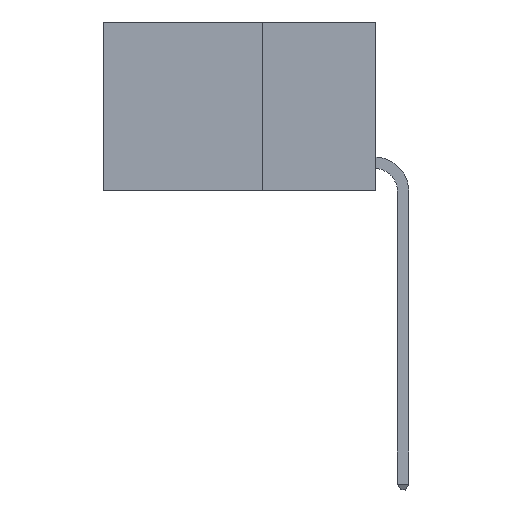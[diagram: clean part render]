
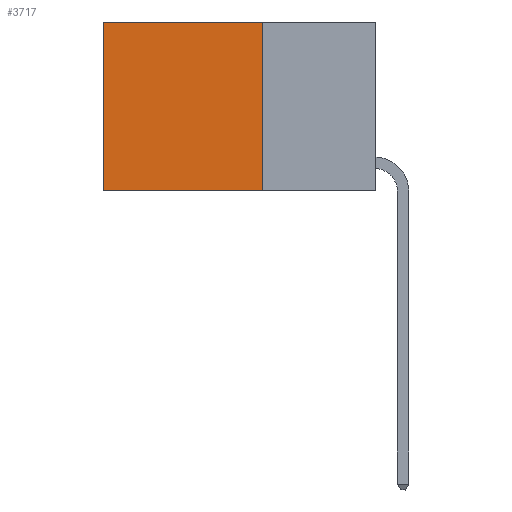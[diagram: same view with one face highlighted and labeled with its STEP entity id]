
A CAD part, left-side view. The second image highlights one B-rep face of the part: STEP entity #3717.
In plain terms, the highlighted planar face has unit normal (-1, 0, 0).
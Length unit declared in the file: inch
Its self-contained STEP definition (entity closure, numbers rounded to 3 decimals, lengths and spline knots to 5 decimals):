
#751 = VECTOR ( 'NONE', #4955, 39.37008 ) ;
#864 = LINE ( 'NONE', #11649, #14065 ) ;
#1375 = DIRECTION ( 'NONE',  ( 0., 0., -1. ) ) ;
#2214 = ORIENTED_EDGE ( 'NONE', *, *, #13067, .T. ) ;
#3605 = DIRECTION ( 'NONE',  ( 0., 0., -1. ) ) ;
#3717 = ADVANCED_FACE ( 'NONE', ( #18977 ), #9644, .F. ) ;
#4151 = CARTESIAN_POINT ( 'NONE',  ( 0.2625, 0.25, -0.37 ) ) ;
#4367 = DIRECTION ( 'NONE',  ( 0., 0., -1. ) ) ;
#4724 = EDGE_LOOP ( 'NONE', ( #7976, #12554, #18352, #2214 ) ) ;
#4955 = DIRECTION ( 'NONE',  ( 0., 1., 0. ) ) ;
#5164 = LINE ( 'NONE', #11529, #751 ) ;
#5405 = AXIS2_PLACEMENT_3D ( 'NONE', #7974, #11284, #1375 ) ;
#5877 = CARTESIAN_POINT ( 'NONE',  ( 0.2625, 0.25, 0. ) ) ;
#7974 = CARTESIAN_POINT ( 'NONE',  ( 0.2625, 0.25, 0. ) ) ;
#7976 = ORIENTED_EDGE ( 'NONE', *, *, #19642, .T. ) ;
#9078 = EDGE_CURVE ( 'NONE', #11327, #13125, #5164, .T. ) ;
#9644 = PLANE ( 'NONE',  #5405 ) ;
#11284 = DIRECTION ( 'NONE',  ( 1., 0., 0. ) ) ;
#11327 = VERTEX_POINT ( 'NONE', #4151 ) ;
#11359 = VERTEX_POINT ( 'NONE', #5877 ) ;
#11529 = CARTESIAN_POINT ( 'NONE',  ( 0.2625, 0.25, -0.37 ) ) ;
#11649 = CARTESIAN_POINT ( 'NONE',  ( 0.2625, 0.25, 0. ) ) ;
#11789 = CARTESIAN_POINT ( 'NONE',  ( 0.2625, 0.6, -0.37 ) ) ;
#12554 = ORIENTED_EDGE ( 'NONE', *, *, #9078, .F. ) ;
#12789 = CARTESIAN_POINT ( 'NONE',  ( 0.2625, 0.6, 0. ) ) ;
#13067 = EDGE_CURVE ( 'NONE', #11359, #14006, #864, .T. ) ;
#13125 = VERTEX_POINT ( 'NONE', #11789 ) ;
#13495 = CARTESIAN_POINT ( 'NONE',  ( 0.2625, 0.6, 0. ) ) ;
#14006 = VERTEX_POINT ( 'NONE', #12789 ) ;
#14065 = VECTOR ( 'NONE', #18256, 39.37008 ) ;
#17472 = CARTESIAN_POINT ( 'NONE',  ( 0.2625, 0.25, 0. ) ) ;
#17619 = LINE ( 'NONE', #13495, #18124 ) ;
#18124 = VECTOR ( 'NONE', #3605, 39.37008 ) ;
#18256 = DIRECTION ( 'NONE',  ( 0., 1., 0. ) ) ;
#18352 = ORIENTED_EDGE ( 'NONE', *, *, #18653, .F. ) ;
#18653 = EDGE_CURVE ( 'NONE', #11359, #11327, #20743, .T. ) ;
#18977 = FACE_OUTER_BOUND ( 'NONE', #4724, .T. ) ;
#19642 = EDGE_CURVE ( 'NONE', #14006, #13125, #17619, .T. ) ;
#19712 = VECTOR ( 'NONE', #4367, 39.37008 ) ;
#20743 = LINE ( 'NONE', #17472, #19712 ) ;
